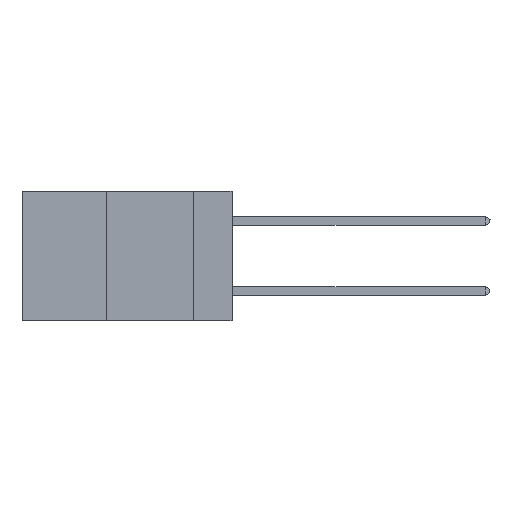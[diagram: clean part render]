
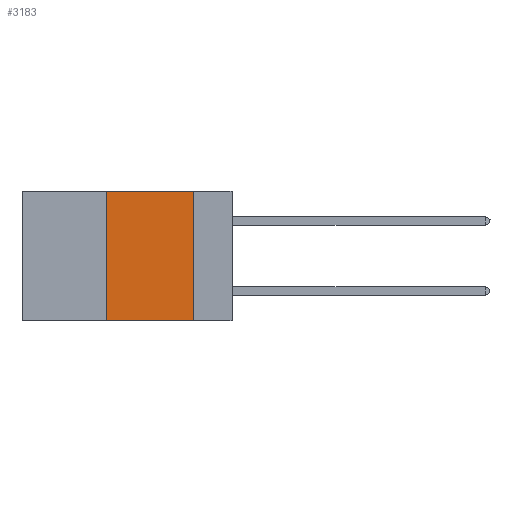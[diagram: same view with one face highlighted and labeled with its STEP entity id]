
A CAD part, left-side view. The second image highlights one B-rep face of the part: STEP entity #3183.
In plain terms, the highlighted planar face has unit normal (-1, 0, 0).
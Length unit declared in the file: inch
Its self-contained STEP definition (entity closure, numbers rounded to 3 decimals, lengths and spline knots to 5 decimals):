
#679 = VERTEX_POINT ( 'NONE', #21529 ) ;
#809 = LINE ( 'NONE', #4203, #14524 ) ;
#1770 = CARTESIAN_POINT ( 'NONE',  ( 0., 0.36, 0. ) ) ;
#1907 = CARTESIAN_POINT ( 'NONE',  ( 0., 0.36, -0.37 ) ) ;
#3183 = ADVANCED_FACE ( 'NONE', ( #10196 ), #11957, .F. ) ;
#4203 = CARTESIAN_POINT ( 'NONE',  ( 0., 0.36, 0. ) ) ;
#4696 = VECTOR ( 'NONE', #26014, 39.37008 ) ;
#4740 = EDGE_CURVE ( 'NONE', #25005, #4793, #12982, .T. ) ;
#4793 = VERTEX_POINT ( 'NONE', #11812 ) ;
#5889 = DIRECTION ( 'NONE',  ( 1., 0., 0. ) ) ;
#6388 = ORIENTED_EDGE ( 'NONE', *, *, #18862, .F. ) ;
#7408 = CARTESIAN_POINT ( 'NONE',  ( 0., 0.11, 0. ) ) ;
#10196 = FACE_OUTER_BOUND ( 'NONE', #12137, .T. ) ;
#10736 = LINE ( 'NONE', #24727, #11372 ) ;
#11372 = VECTOR ( 'NONE', #18667, 39.37008 ) ;
#11812 = CARTESIAN_POINT ( 'NONE',  ( 0., 0.11, 0. ) ) ;
#11957 = PLANE ( 'NONE',  #13450 ) ;
#12137 = EDGE_LOOP ( 'NONE', ( #6388, #23207, #13814, #22474 ) ) ;
#12982 = LINE ( 'NONE', #13613, #4696 ) ;
#13450 = AXIS2_PLACEMENT_3D ( 'NONE', #13845, #5889, #13935 ) ;
#13613 = CARTESIAN_POINT ( 'NONE',  ( 0., 0.6, 0. ) ) ;
#13814 = ORIENTED_EDGE ( 'NONE', *, *, #19685, .F. ) ;
#13845 = CARTESIAN_POINT ( 'NONE',  ( 0., 0.6, 0. ) ) ;
#13935 = DIRECTION ( 'NONE',  ( 0., 0., -1. ) ) ;
#14524 = VECTOR ( 'NONE', #20435, 39.37008 ) ;
#15548 = EDGE_CURVE ( 'NONE', #23097, #679, #10736, .T. ) ;
#17618 = VECTOR ( 'NONE', #21727, 39.37008 ) ;
#18667 = DIRECTION ( 'NONE',  ( 0., -1., 0. ) ) ;
#18862 = EDGE_CURVE ( 'NONE', #4793, #679, #24628, .T. ) ;
#19685 = EDGE_CURVE ( 'NONE', #23097, #25005, #809, .T. ) ;
#20435 = DIRECTION ( 'NONE',  ( 0., 0., 1. ) ) ;
#21529 = CARTESIAN_POINT ( 'NONE',  ( 0., 0.11, -0.37 ) ) ;
#21727 = DIRECTION ( 'NONE',  ( 0., 0., -1. ) ) ;
#22474 = ORIENTED_EDGE ( 'NONE', *, *, #15548, .T. ) ;
#23097 = VERTEX_POINT ( 'NONE', #1907 ) ;
#23207 = ORIENTED_EDGE ( 'NONE', *, *, #4740, .F. ) ;
#24628 = LINE ( 'NONE', #7408, #17618 ) ;
#24727 = CARTESIAN_POINT ( 'NONE',  ( 0., 0.6, -0.37 ) ) ;
#25005 = VERTEX_POINT ( 'NONE', #1770 ) ;
#26014 = DIRECTION ( 'NONE',  ( 0., -1., 0. ) ) ;
